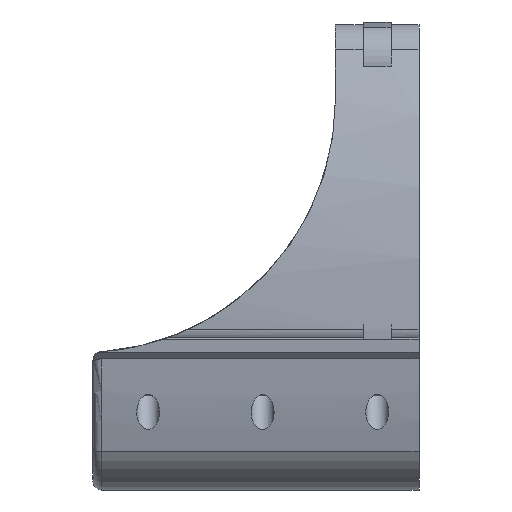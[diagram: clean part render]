
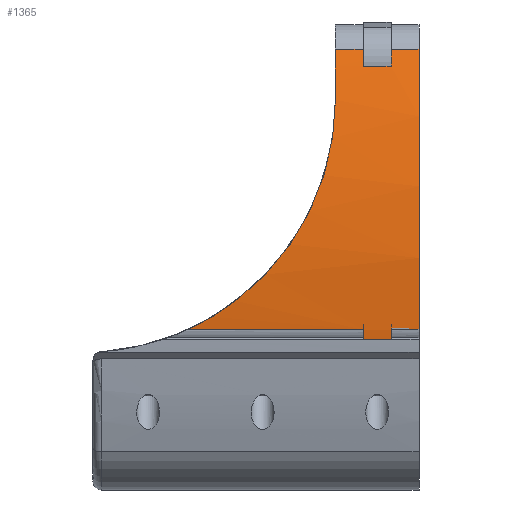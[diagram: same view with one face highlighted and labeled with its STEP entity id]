
A CAD part, left-side view. The second image highlights one B-rep face of the part: STEP entity #1365.
In plain terms, the highlighted cylindrical face has radius 200.536 mm (diameter 401.073 mm), a partial arc.
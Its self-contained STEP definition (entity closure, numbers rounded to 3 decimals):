
#145=FACE_OUTER_BOUND('',#241,.T.);
#241=EDGE_LOOP('',(#1167,#1168,#1169,#1170,#1171,#1172,#1173,#1174,#1175,
#1176,#1177,#1178,#1179,#1180,#1181));
#287=B_SPLINE_CURVE_WITH_KNOTS('',3,(#2622,#2623,#2624,#2625,#2626,#2627,
#2628,#2629,#2630,#2631,#2632,#2633,#2634,#2635),.UNSPECIFIED.,.F.,.F.,
(4,2,2,2,2,2,4),(4.101,4.651,6.976,9.301,
11.505,13.709,14.348),.UNSPECIFIED.);
#346=LINE('',#2683,#442);
#354=LINE('',#2709,#450);
#358=LINE('',#2724,#454);
#359=LINE('',#2728,#455);
#360=LINE('',#2729,#456);
#361=LINE('',#2731,#457);
#362=LINE('',#2734,#458);
#363=LINE('',#2737,#459);
#442=VECTOR('',#1840,10.);
#450=VECTOR('',#1864,10.);
#454=VECTOR('',#1880,10.);
#455=VECTOR('',#1883,10.);
#456=VECTOR('',#1884,10.);
#457=VECTOR('',#1885,10.);
#458=VECTOR('',#1888,10.);
#459=VECTOR('',#1891,10.);
#529=CIRCLE('',#1513,200.536);
#540=CIRCLE('',#1530,200.536);
#541=CIRCLE('',#1532,200.536);
#542=CIRCLE('',#1533,200.536);
#543=CIRCLE('',#1534,200.536);
#544=CIRCLE('',#1535,200.536);
#636=VERTEX_POINT('',#2620);
#637=VERTEX_POINT('',#2621);
#640=VERTEX_POINT('',#2671);
#644=VERTEX_POINT('',#2681);
#653=VERTEX_POINT('',#2707);
#654=VERTEX_POINT('',#2708);
#657=VERTEX_POINT('',#2716);
#658=VERTEX_POINT('',#2721);
#659=VERTEX_POINT('',#2723);
#660=VERTEX_POINT('',#2725);
#661=VERTEX_POINT('',#2727);
#662=VERTEX_POINT('',#2730);
#663=VERTEX_POINT('',#2732);
#664=VERTEX_POINT('',#2735);
#806=EDGE_CURVE('',#636,#637,#287,.T.);
#810=EDGE_CURVE('',#640,#636,#529,.T.);
#816=EDGE_CURVE('',#644,#637,#346,.T.);
#828=EDGE_CURVE('',#653,#654,#354,.T.);
#834=EDGE_CURVE('',#657,#653,#540,.T.);
#835=EDGE_CURVE('',#644,#658,#541,.T.);
#836=EDGE_CURVE('',#659,#658,#358,.T.);
#837=EDGE_CURVE('',#659,#660,#542,.T.);
#838=EDGE_CURVE('',#660,#661,#359,.T.);
#839=EDGE_CURVE('',#660,#661,#360,.T.);
#840=EDGE_CURVE('',#662,#660,#361,.T.);
#841=EDGE_CURVE('',#662,#663,#543,.T.);
#842=EDGE_CURVE('',#663,#657,#362,.T.);
#843=EDGE_CURVE('',#654,#664,#544,.T.);
#844=EDGE_CURVE('',#664,#640,#363,.T.);
#1167=ORIENTED_EDGE('',*,*,#806,.T.);
#1168=ORIENTED_EDGE('',*,*,#816,.F.);
#1169=ORIENTED_EDGE('',*,*,#835,.T.);
#1170=ORIENTED_EDGE('',*,*,#836,.F.);
#1171=ORIENTED_EDGE('',*,*,#837,.T.);
#1172=ORIENTED_EDGE('',*,*,#838,.T.);
#1173=ORIENTED_EDGE('',*,*,#839,.F.);
#1174=ORIENTED_EDGE('',*,*,#840,.F.);
#1175=ORIENTED_EDGE('',*,*,#841,.T.);
#1176=ORIENTED_EDGE('',*,*,#842,.T.);
#1177=ORIENTED_EDGE('',*,*,#834,.T.);
#1178=ORIENTED_EDGE('',*,*,#828,.T.);
#1179=ORIENTED_EDGE('',*,*,#843,.T.);
#1180=ORIENTED_EDGE('',*,*,#844,.T.);
#1181=ORIENTED_EDGE('',*,*,#810,.T.);
#1301=CYLINDRICAL_SURFACE('',#1531,200.536);
#1365=ADVANCED_FACE('',(#145),#1301,.T.);
#1513=AXIS2_PLACEMENT_3D('',#2672,#1827,#1828);
#1530=AXIS2_PLACEMENT_3D('',#2719,#1874,#1875);
#1531=AXIS2_PLACEMENT_3D('',#2720,#1876,#1877);
#1532=AXIS2_PLACEMENT_3D('',#2722,#1878,#1879);
#1533=AXIS2_PLACEMENT_3D('',#2726,#1881,#1882);
#1534=AXIS2_PLACEMENT_3D('',#2733,#1886,#1887);
#1535=AXIS2_PLACEMENT_3D('',#2736,#1889,#1890);
#1827=DIRECTION('center_axis',(0.,-1.,0.));
#1828=DIRECTION('ref_axis',(-0.953,0.,-0.304));
#1840=DIRECTION('',(0.,1.,0.));
#1864=DIRECTION('',(0.,1.,0.));
#1874=DIRECTION('center_axis',(0.,-1.,0.));
#1875=DIRECTION('ref_axis',(-0.953,0.,-0.304));
#1876=DIRECTION('center_axis',(0.,1.,0.));
#1877=DIRECTION('ref_axis',(-0.953,0.,-0.304));
#1878=DIRECTION('center_axis',(0.,-1.,0.));
#1879=DIRECTION('ref_axis',(-0.953,0.,-0.304));
#1880=DIRECTION('',(0.,1.,0.));
#1881=DIRECTION('center_axis',(0.,1.,0.));
#1882=DIRECTION('ref_axis',(-0.953,0.,-0.304));
#1883=DIRECTION('',(0.,1.,0.));
#1884=DIRECTION('',(0.,1.,0.));
#1885=DIRECTION('',(0.,1.,0.));
#1886=DIRECTION('center_axis',(0.,1.,0.));
#1887=DIRECTION('ref_axis',(-0.953,0.,-0.304));
#1888=DIRECTION('',(0.,1.,0.));
#1889=DIRECTION('center_axis',(0.,1.,0.));
#1890=DIRECTION('ref_axis',(-0.953,0.,-0.304));
#1891=DIRECTION('',(0.,1.,0.));
#2620=CARTESIAN_POINT('',(-19.937,30.,116.5));
#2621=CARTESIAN_POINT('',(-30.123,83.201,33.952));
#2622=CARTESIAN_POINT('Ctrl Pts',(-19.937,30.,116.5));
#2623=CARTESIAN_POINT('Ctrl Pts',(-20.556,30.,114.704));
#2624=CARTESIAN_POINT('Ctrl Pts',(-21.148,30.053,112.902));
#2625=CARTESIAN_POINT('Ctrl Pts',(-24.101,30.617,103.466));
#2626=CARTESIAN_POINT('Ctrl Pts',(-25.999,32.06,95.761));
#2627=CARTESIAN_POINT('Ctrl Pts',(-28.793,36.905,80.934));
#2628=CARTESIAN_POINT('Ctrl Pts',(-29.694,40.308,73.813));
#2629=CARTESIAN_POINT('Ctrl Pts',(-30.714,48.481,61.161));
#2630=CARTESIAN_POINT('Ctrl Pts',(-30.889,53.306,55.354));
#2631=CARTESIAN_POINT('Ctrl Pts',(-30.838,64.358,45.049));
#2632=CARTESIAN_POINT('Ctrl Pts',(-30.616,70.586,40.551));
#2633=CARTESIAN_POINT('Ctrl Pts',(-30.28,79.211,35.851));
#2634=CARTESIAN_POINT('Ctrl Pts',(-30.202,81.19,34.864));
#2635=CARTESIAN_POINT('Ctrl Pts',(-30.123,83.201,33.952));
#2671=CARTESIAN_POINT('',(-12.652,30.,134.709));
#2672=CARTESIAN_POINT('Origin',(169.67,30.,51.202));
#2681=CARTESIAN_POINT('',(-30.123,20.,33.952));
#2683=CARTESIAN_POINT('',(-30.123,20.,33.952));
#2707=CARTESIAN_POINT('',(-15.347,10.,128.555));
#2708=CARTESIAN_POINT('',(-15.347,20.,128.555));
#2709=CARTESIAN_POINT('',(-15.347,0.,128.555));
#2716=CARTESIAN_POINT('',(-12.652,10.,134.709));
#2719=CARTESIAN_POINT('Origin',(169.67,10.,51.202));
#2720=CARTESIAN_POINT('Origin',(169.67,0.,51.202));
#2721=CARTESIAN_POINT('',(-29.807,20.,30.618));
#2722=CARTESIAN_POINT('Origin',(169.67,20.,51.202));
#2723=CARTESIAN_POINT('',(-29.807,9.982,30.618));
#2724=CARTESIAN_POINT('',(-29.807,0.,30.618));
#2725=CARTESIAN_POINT('',(-30.123,9.982,33.952));
#2726=CARTESIAN_POINT('Origin',(169.67,9.982,51.202));
#2727=CARTESIAN_POINT('',(-30.123,10.,33.952));
#2728=CARTESIAN_POINT('',(-30.123,20.,33.952));
#2729=CARTESIAN_POINT('',(-30.123,20.,33.952));
#2730=CARTESIAN_POINT('',(-30.123,0.,33.952));
#2731=CARTESIAN_POINT('',(-30.123,20.,33.952));
#2732=CARTESIAN_POINT('',(-12.652,0.,134.709));
#2733=CARTESIAN_POINT('Origin',(169.67,0.,51.202));
#2734=CARTESIAN_POINT('',(-12.652,0.,134.709));
#2735=CARTESIAN_POINT('',(-12.652,20.,134.709));
#2736=CARTESIAN_POINT('Origin',(169.67,20.,51.202));
#2737=CARTESIAN_POINT('',(-12.652,0.,134.709));
